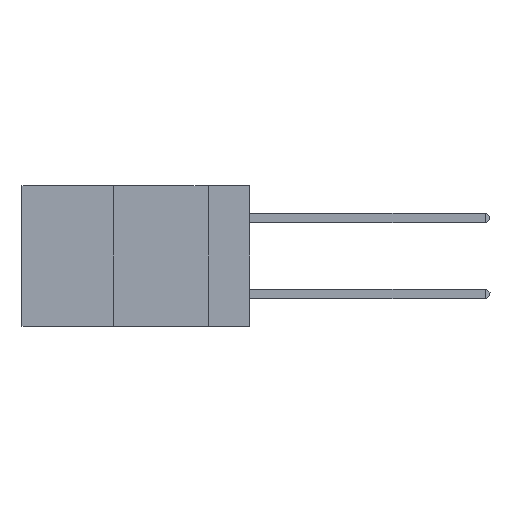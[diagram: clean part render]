
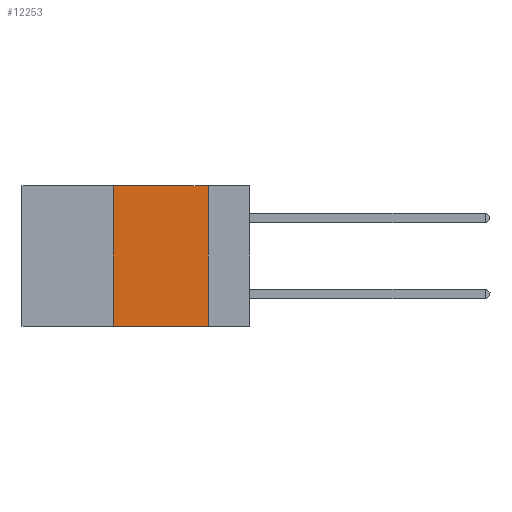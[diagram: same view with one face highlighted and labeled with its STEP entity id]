
A CAD part, left-side view. The second image highlights one B-rep face of the part: STEP entity #12253.
In plain terms, the highlighted planar face has unit normal (-1, 0, 0).
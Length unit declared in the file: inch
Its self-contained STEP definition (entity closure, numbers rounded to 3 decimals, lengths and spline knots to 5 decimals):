
#61 = VECTOR ( 'NONE', #6491, 39.37008 ) ;
#86 = CARTESIAN_POINT ( 'NONE',  ( 0., 0.11, -0.37 ) ) ;
#710 = LINE ( 'NONE', #1828, #1615 ) ;
#1206 = ORIENTED_EDGE ( 'NONE', *, *, #9928, .F. ) ;
#1395 = DIRECTION ( 'NONE',  ( 1., 0., 0. ) ) ;
#1615 = VECTOR ( 'NONE', #2973, 39.37008 ) ;
#1648 = VERTEX_POINT ( 'NONE', #7042 ) ;
#1818 = EDGE_CURVE ( 'NONE', #12219, #9519, #710, .T. ) ;
#1828 = CARTESIAN_POINT ( 'NONE',  ( 0., 0.11, 0. ) ) ;
#2077 = EDGE_CURVE ( 'NONE', #1648, #12219, #8776, .T. ) ;
#2742 = ORIENTED_EDGE ( 'NONE', *, *, #1818, .F. ) ;
#2758 = AXIS2_PLACEMENT_3D ( 'NONE', #5085, #1395, #4925 ) ;
#2851 = CARTESIAN_POINT ( 'NONE',  ( 0., 0.6, -0.37 ) ) ;
#2973 = DIRECTION ( 'NONE',  ( 0., 0., -1. ) ) ;
#3151 = ORIENTED_EDGE ( 'NONE', *, *, #11725, .T. ) ;
#4925 = DIRECTION ( 'NONE',  ( 0., 0., -1. ) ) ;
#5085 = CARTESIAN_POINT ( 'NONE',  ( 0., 0.6, 0. ) ) ;
#5796 = EDGE_LOOP ( 'NONE', ( #2742, #12398, #1206, #3151 ) ) ;
#6199 = CARTESIAN_POINT ( 'NONE',  ( 0., 0.36, -0.37 ) ) ;
#6491 = DIRECTION ( 'NONE',  ( 0., -1., 0. ) ) ;
#6597 = VERTEX_POINT ( 'NONE', #6199 ) ;
#7042 = CARTESIAN_POINT ( 'NONE',  ( 0., 0.36, 0. ) ) ;
#7686 = VECTOR ( 'NONE', #12038, 39.37008 ) ;
#8776 = LINE ( 'NONE', #14432, #7686 ) ;
#8918 = LINE ( 'NONE', #11361, #11789 ) ;
#9465 = CARTESIAN_POINT ( 'NONE',  ( 0., 0.11, 0. ) ) ;
#9519 = VERTEX_POINT ( 'NONE', #86 ) ;
#9928 = EDGE_CURVE ( 'NONE', #6597, #1648, #8918, .T. ) ;
#11193 = FACE_OUTER_BOUND ( 'NONE', #5796, .T. ) ;
#11361 = CARTESIAN_POINT ( 'NONE',  ( 0., 0.36, 0. ) ) ;
#11725 = EDGE_CURVE ( 'NONE', #6597, #9519, #12829, .T. ) ;
#11789 = VECTOR ( 'NONE', #12423, 39.37008 ) ;
#11797 = PLANE ( 'NONE',  #2758 ) ;
#12038 = DIRECTION ( 'NONE',  ( 0., -1., 0. ) ) ;
#12219 = VERTEX_POINT ( 'NONE', #9465 ) ;
#12253 = ADVANCED_FACE ( 'NONE', ( #11193 ), #11797, .F. ) ;
#12398 = ORIENTED_EDGE ( 'NONE', *, *, #2077, .F. ) ;
#12423 = DIRECTION ( 'NONE',  ( 0., 0., 1. ) ) ;
#12829 = LINE ( 'NONE', #2851, #61 ) ;
#14432 = CARTESIAN_POINT ( 'NONE',  ( 0., 0.6, 0. ) ) ;
